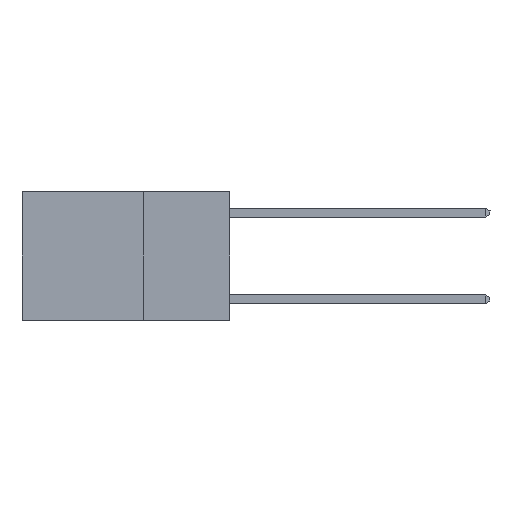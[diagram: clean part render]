
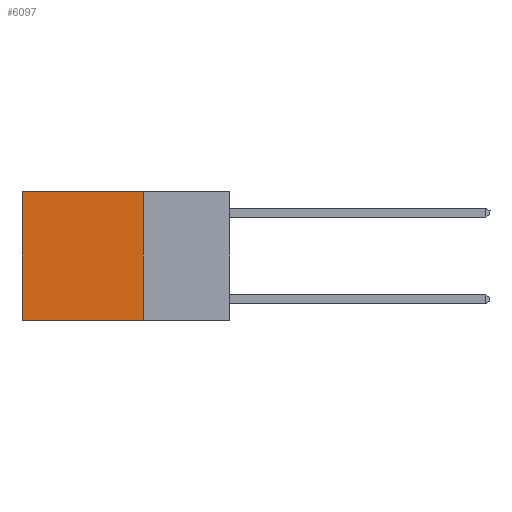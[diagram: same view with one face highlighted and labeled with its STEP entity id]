
A CAD part, left-side view. The second image highlights one B-rep face of the part: STEP entity #6097.
In plain terms, the highlighted planar face has unit normal (-1, 0, 0).
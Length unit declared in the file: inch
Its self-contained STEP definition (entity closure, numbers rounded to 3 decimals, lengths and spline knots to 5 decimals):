
#67 = ORIENTED_EDGE ( 'NONE', *, *, #9090, .T. ) ;
#138 = EDGE_CURVE ( 'NONE', #4284, #11733, #14590, .T. ) ;
#242 = DIRECTION ( 'NONE',  ( 0., 1., 0. ) ) ;
#1058 = DIRECTION ( 'NONE',  ( 0., 0., -1. ) ) ;
#1080 = ORIENTED_EDGE ( 'NONE', *, *, #14569, .F. ) ;
#1388 = DIRECTION ( 'NONE',  ( 0., 0., -1. ) ) ;
#1796 = CARTESIAN_POINT ( 'NONE',  ( 0.2625, 0.6, -0.37 ) ) ;
#3616 = FACE_OUTER_BOUND ( 'NONE', #6291, .T. ) ;
#4014 = CARTESIAN_POINT ( 'NONE',  ( 0.2625, 0.6, 0. ) ) ;
#4132 = VECTOR ( 'NONE', #5907, 39.37008 ) ;
#4284 = VERTEX_POINT ( 'NONE', #5564 ) ;
#5491 = ORIENTED_EDGE ( 'NONE', *, *, #15683, .T. ) ;
#5564 = CARTESIAN_POINT ( 'NONE',  ( 0.2625, 0.25, -0.37 ) ) ;
#5907 = DIRECTION ( 'NONE',  ( 0., 0., -1. ) ) ;
#5915 = VECTOR ( 'NONE', #1388, 39.37008 ) ;
#6046 = VERTEX_POINT ( 'NONE', #8796 ) ;
#6097 = ADVANCED_FACE ( 'NONE', ( #3616 ), #6304, .F. ) ;
#6291 = EDGE_LOOP ( 'NONE', ( #5491, #8821, #1080, #67 ) ) ;
#6304 = PLANE ( 'NONE',  #13727 ) ;
#6847 = DIRECTION ( 'NONE',  ( 0., 1., 0. ) ) ;
#7437 = VECTOR ( 'NONE', #242, 39.37008 ) ;
#8487 = CARTESIAN_POINT ( 'NONE',  ( 0.2625, 0.25, 0. ) ) ;
#8796 = CARTESIAN_POINT ( 'NONE',  ( 0.2625, 0.6, 0. ) ) ;
#8821 = ORIENTED_EDGE ( 'NONE', *, *, #138, .F. ) ;
#8917 = DIRECTION ( 'NONE',  ( 1., 0., 0. ) ) ;
#9090 = EDGE_CURVE ( 'NONE', #13834, #6046, #12676, .T. ) ;
#10562 = CARTESIAN_POINT ( 'NONE',  ( 0.2625, 0.25, -0.37 ) ) ;
#11379 = LINE ( 'NONE', #8487, #4132 ) ;
#11733 = VERTEX_POINT ( 'NONE', #1796 ) ;
#12676 = LINE ( 'NONE', #13192, #15610 ) ;
#12696 = LINE ( 'NONE', #4014, #5915 ) ;
#13192 = CARTESIAN_POINT ( 'NONE',  ( 0.2625, 0.25, 0. ) ) ;
#13727 = AXIS2_PLACEMENT_3D ( 'NONE', #16439, #8917, #1058 ) ;
#13834 = VERTEX_POINT ( 'NONE', #14755 ) ;
#14569 = EDGE_CURVE ( 'NONE', #13834, #4284, #11379, .T. ) ;
#14590 = LINE ( 'NONE', #10562, #7437 ) ;
#14755 = CARTESIAN_POINT ( 'NONE',  ( 0.2625, 0.25, 0. ) ) ;
#15610 = VECTOR ( 'NONE', #6847, 39.37008 ) ;
#15683 = EDGE_CURVE ( 'NONE', #6046, #11733, #12696, .T. ) ;
#16439 = CARTESIAN_POINT ( 'NONE',  ( 0.2625, 0.25, 0. ) ) ;
